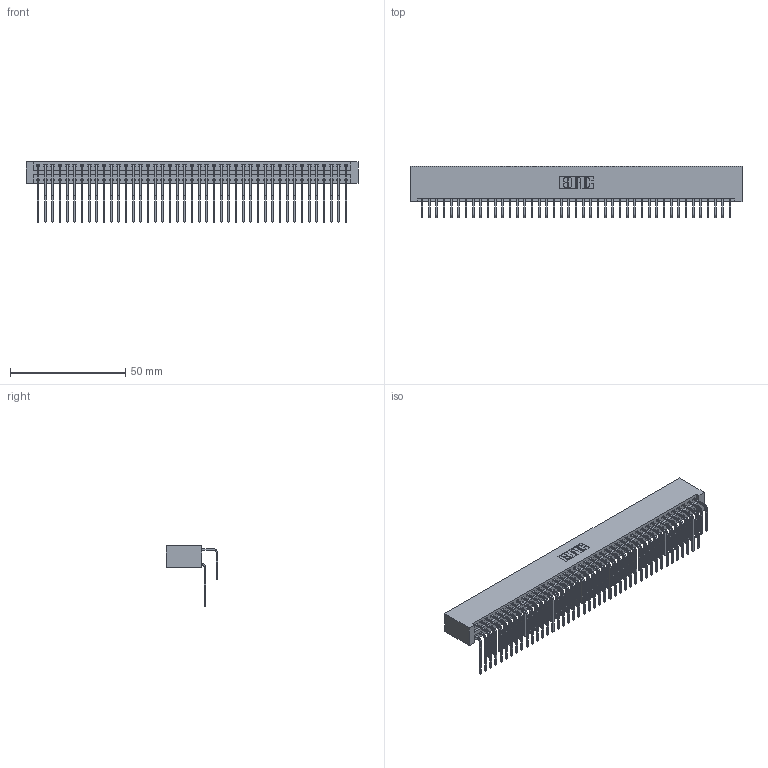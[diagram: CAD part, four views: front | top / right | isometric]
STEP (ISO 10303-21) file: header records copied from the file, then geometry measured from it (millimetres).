
FILE_DESCRIPTION (( 'STEP AP203' ), '1' );
FILE_NAME ('346-086-558-201.STEP', '2018-08-29T23:10:51', ( '' ), ( '' ), 'SwSTEP 2.0', 'SolidWorks 2016', '' );
FILE_SCHEMA (( 'CONFIG_CONTROL_DESIGN' ));
Length unit declared in the file: inch
Products named in the file (4): 345-292-001_558 Tail - 2; 346-086-558-201; 346 Part_No Mounting Lugs; 345-292-001_558 559 Tail - 1
Assembly tree (87 placements, depth 2):
  346-086-558-201
    346 Part_No Mounting Lugs
    345-292-001_558 559 Tail - 1  x43
    345-292-001_558 Tail - 2  x43
Bounding box: 143.76 x 22.16 x 26.16 mm (x, y, z)
Volume: 15095.9 mm3; surface area: 23309.3 mm2
Topology: 87 solids, 87 shells, 4758 faces, 14151 edges, 9318 vertices
Faces by surface type: plane 3254, cylinder 1504
Entity records: 29435 total; most frequent: CARTESIAN_POINT 4899, ORIENTED_EDGE 4782, DIRECTION 4335, EDGE_CURVE 2391, LINE 2055, VECTOR 2055, VERTEX_POINT 1590, AXIS2_PLACEMENT_3D 1140
